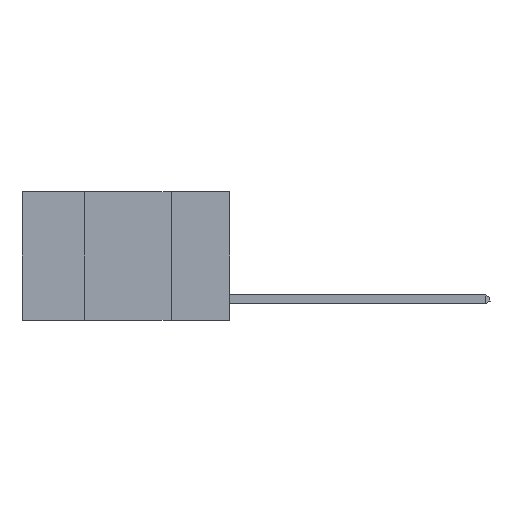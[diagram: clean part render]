
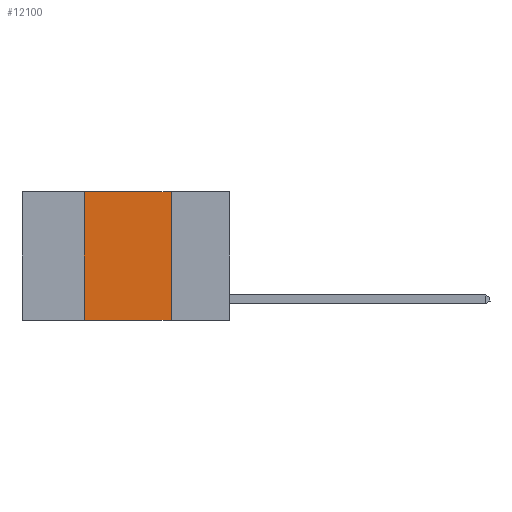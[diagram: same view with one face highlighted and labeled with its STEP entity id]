
A CAD part, left-side view. The second image highlights one B-rep face of the part: STEP entity #12100.
In plain terms, the highlighted planar face has unit normal (-1, 0, 0).
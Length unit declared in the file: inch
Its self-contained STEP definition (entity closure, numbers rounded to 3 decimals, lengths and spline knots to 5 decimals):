
#855 = FACE_OUTER_BOUND ( 'NONE', #8227, .T. ) ;
#1061 = DIRECTION ( 'NONE',  ( 0., -1., 0. ) ) ;
#1441 = DIRECTION ( 'NONE',  ( 0., 0., -1. ) ) ;
#1537 = CARTESIAN_POINT ( 'NONE',  ( 0., 0.42, 0. ) ) ;
#1561 = ORIENTED_EDGE ( 'NONE', *, *, #7181, .F. ) ;
#2101 = EDGE_CURVE ( 'NONE', #11728, #9171, #2517, .T. ) ;
#2333 = CARTESIAN_POINT ( 'NONE',  ( 0., 0.42, 0. ) ) ;
#2517 = LINE ( 'NONE', #6270, #5078 ) ;
#3137 = VERTEX_POINT ( 'NONE', #7631 ) ;
#4177 = ORIENTED_EDGE ( 'NONE', *, *, #2101, .F. ) ;
#5078 = VECTOR ( 'NONE', #10994, 39.37008 ) ;
#5547 = CARTESIAN_POINT ( 'NONE',  ( 0., 0.17, 0. ) ) ;
#5703 = LINE ( 'NONE', #7864, #7267 ) ;
#6270 = CARTESIAN_POINT ( 'NONE',  ( 0., 0.6, 0. ) ) ;
#6625 = PLANE ( 'NONE',  #6931 ) ;
#6931 = AXIS2_PLACEMENT_3D ( 'NONE', #9365, #11276, #12286 ) ;
#7101 = CARTESIAN_POINT ( 'NONE',  ( 0., 0.17, -0.37 ) ) ;
#7181 = EDGE_CURVE ( 'NONE', #9171, #10331, #11117, .T. ) ;
#7267 = VECTOR ( 'NONE', #1061, 39.37008 ) ;
#7316 = EDGE_CURVE ( 'NONE', #3137, #10331, #5703, .T. ) ;
#7631 = CARTESIAN_POINT ( 'NONE',  ( 0., 0.42, -0.37 ) ) ;
#7864 = CARTESIAN_POINT ( 'NONE',  ( 0., 0.6, -0.37 ) ) ;
#8157 = ORIENTED_EDGE ( 'NONE', *, *, #7316, .T. ) ;
#8227 = EDGE_LOOP ( 'NONE', ( #1561, #4177, #10417, #8157 ) ) ;
#9171 = VERTEX_POINT ( 'NONE', #5547 ) ;
#9365 = CARTESIAN_POINT ( 'NONE',  ( 0., 0.6, 0. ) ) ;
#9504 = EDGE_CURVE ( 'NONE', #3137, #11728, #10257, .T. ) ;
#9928 = VECTOR ( 'NONE', #1441, 39.37008 ) ;
#10171 = CARTESIAN_POINT ( 'NONE',  ( 0., 0.17, 0. ) ) ;
#10257 = LINE ( 'NONE', #1537, #11935 ) ;
#10331 = VERTEX_POINT ( 'NONE', #7101 ) ;
#10417 = ORIENTED_EDGE ( 'NONE', *, *, #9504, .F. ) ;
#10994 = DIRECTION ( 'NONE',  ( 0., -1., 0. ) ) ;
#11117 = LINE ( 'NONE', #10171, #9928 ) ;
#11276 = DIRECTION ( 'NONE',  ( 1., 0., 0. ) ) ;
#11728 = VERTEX_POINT ( 'NONE', #2333 ) ;
#11935 = VECTOR ( 'NONE', #12273, 39.37008 ) ;
#12100 = ADVANCED_FACE ( 'NONE', ( #855 ), #6625, .F. ) ;
#12273 = DIRECTION ( 'NONE',  ( 0., 0., 1. ) ) ;
#12286 = DIRECTION ( 'NONE',  ( 0., 0., -1. ) ) ;
